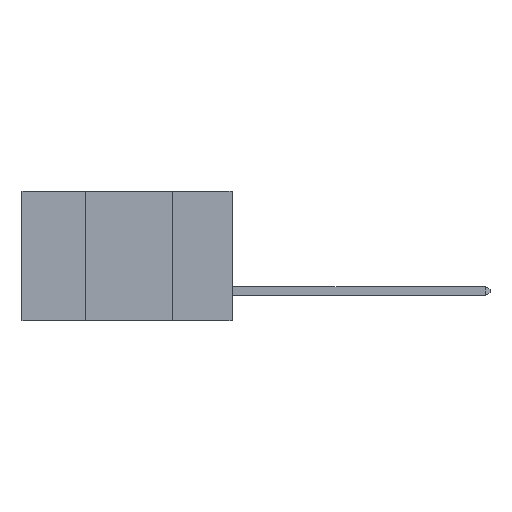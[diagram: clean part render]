
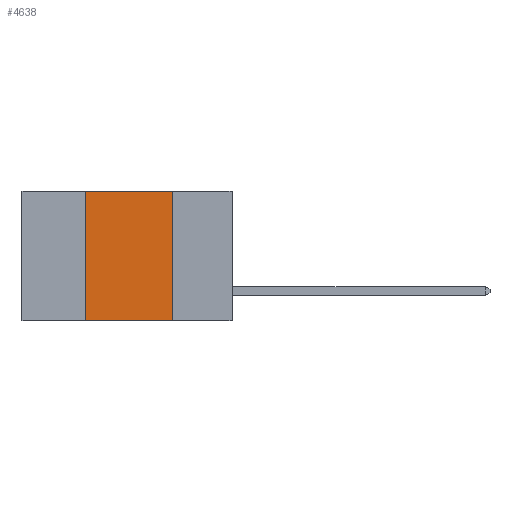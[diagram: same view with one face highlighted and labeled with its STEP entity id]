
A CAD part, left-side view. The second image highlights one B-rep face of the part: STEP entity #4638.
In plain terms, the highlighted planar face has unit normal (-1, 0, 0).
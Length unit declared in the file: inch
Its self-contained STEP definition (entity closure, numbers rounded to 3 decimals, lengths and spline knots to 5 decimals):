
#137 = ORIENTED_EDGE ( 'NONE', *, *, #5661, .F. ) ;
#160 = VERTEX_POINT ( 'NONE', #304 ) ;
#304 = CARTESIAN_POINT ( 'NONE',  ( 0., 0.17, -0.37 ) ) ;
#1032 = DIRECTION ( 'NONE',  ( 0., -1., 0. ) ) ;
#1258 = EDGE_CURVE ( 'NONE', #2553, #10429, #10694, .T. ) ;
#1725 = DIRECTION ( 'NONE',  ( 1., 0., 0. ) ) ;
#2399 = CARTESIAN_POINT ( 'NONE',  ( 0., 0.17, 0. ) ) ;
#2553 = VERTEX_POINT ( 'NONE', #10529 ) ;
#2853 = VECTOR ( 'NONE', #4708, 39.37008 ) ;
#3620 = EDGE_CURVE ( 'NONE', #10469, #160, #10065, .T. ) ;
#4131 = VECTOR ( 'NONE', #11801, 39.37008 ) ;
#4224 = ORIENTED_EDGE ( 'NONE', *, *, #4610, .F. ) ;
#4334 = AXIS2_PLACEMENT_3D ( 'NONE', #11612, #1725, #8722 ) ;
#4610 = EDGE_CURVE ( 'NONE', #10429, #160, #6816, .T. ) ;
#4638 = ADVANCED_FACE ( 'NONE', ( #8664 ), #6132, .F. ) ;
#4670 = ORIENTED_EDGE ( 'NONE', *, *, #3620, .T. ) ;
#4708 = DIRECTION ( 'NONE',  ( 0., -1., 0. ) ) ;
#4732 = CARTESIAN_POINT ( 'NONE',  ( 0., 0.6, -0.37 ) ) ;
#5661 = EDGE_CURVE ( 'NONE', #10469, #2553, #9601, .T. ) ;
#5782 = DIRECTION ( 'NONE',  ( 0., 0., 1. ) ) ;
#5917 = VECTOR ( 'NONE', #1032, 39.37008 ) ;
#6132 = PLANE ( 'NONE',  #4334 ) ;
#6816 = LINE ( 'NONE', #2399, #4131 ) ;
#6938 = VECTOR ( 'NONE', #5782, 39.37008 ) ;
#7401 = CARTESIAN_POINT ( 'NONE',  ( 0., 0.6, 0. ) ) ;
#7553 = CARTESIAN_POINT ( 'NONE',  ( 0., 0.42, 0. ) ) ;
#8060 = ORIENTED_EDGE ( 'NONE', *, *, #1258, .F. ) ;
#8664 = FACE_OUTER_BOUND ( 'NONE', #11045, .T. ) ;
#8722 = DIRECTION ( 'NONE',  ( 0., 0., -1. ) ) ;
#9524 = CARTESIAN_POINT ( 'NONE',  ( 0., 0.17, 0. ) ) ;
#9601 = LINE ( 'NONE', #7553, #6938 ) ;
#10065 = LINE ( 'NONE', #4732, #2853 ) ;
#10429 = VERTEX_POINT ( 'NONE', #9524 ) ;
#10469 = VERTEX_POINT ( 'NONE', #11364 ) ;
#10529 = CARTESIAN_POINT ( 'NONE',  ( 0., 0.42, 0. ) ) ;
#10694 = LINE ( 'NONE', #7401, #5917 ) ;
#11045 = EDGE_LOOP ( 'NONE', ( #4224, #8060, #137, #4670 ) ) ;
#11364 = CARTESIAN_POINT ( 'NONE',  ( 0., 0.42, -0.37 ) ) ;
#11612 = CARTESIAN_POINT ( 'NONE',  ( 0., 0.6, 0. ) ) ;
#11801 = DIRECTION ( 'NONE',  ( 0., 0., -1. ) ) ;
